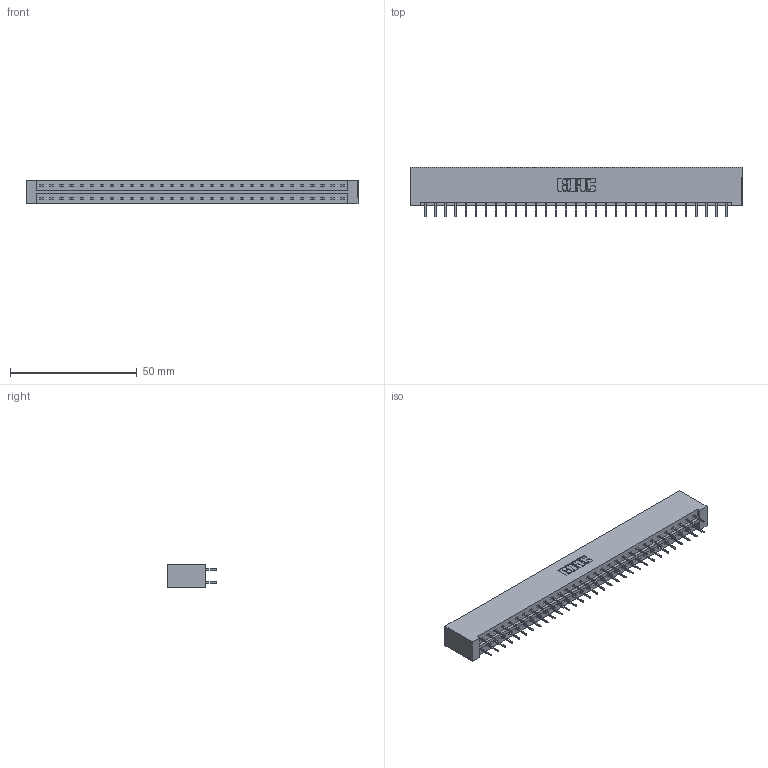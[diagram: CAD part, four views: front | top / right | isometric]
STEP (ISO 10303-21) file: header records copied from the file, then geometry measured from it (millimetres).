
FILE_DESCRIPTION (( 'STEP AP203' ), '1' );
FILE_NAME ('333-062-524-201.STEP', '2018-08-04T08:21:04', ( '' ), ( '' ), 'SwSTEP 2.0', 'SolidWorks 2016', '' );
FILE_SCHEMA (( 'CONFIG_CONTROL_DESIGN' ));
Length unit declared in the file: inch
Products named in the file (3): 333 Part_Lugless; 345-292-001_345-293-124; 333-062-524-201
Assembly tree (63 placements, depth 2):
  333-062-524-201
    333 Part_Lugless
    345-292-001_345-293-124  x62
Bounding box: 131.09 x 19.69 x 9.4 mm (x, y, z)
Volume: 13819 mm3; surface area: 15962.1 mm2
Topology: 63 solids, 63 shells, 3578 faces, 10145 edges, 6514 vertices
Faces by surface type: plane 2670, cylinder 908
Entity records: 21163 total; most frequent: CARTESIAN_POINT 3518, ORIENTED_EDGE 3454, DIRECTION 3019, EDGE_CURVE 1727, VECTOR 1611, LINE 1611, VERTEX_POINT 1146, AXIS2_PLACEMENT_3D 704
